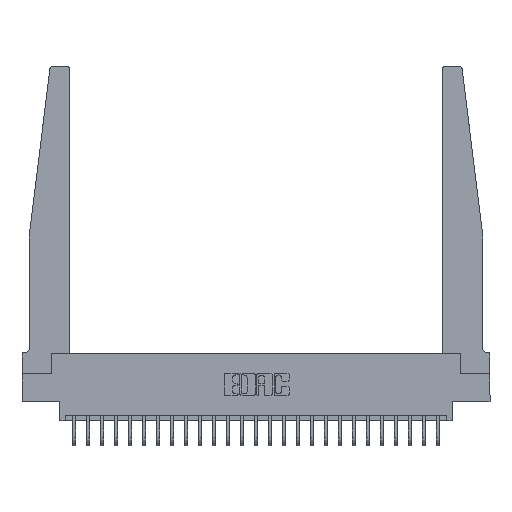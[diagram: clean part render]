
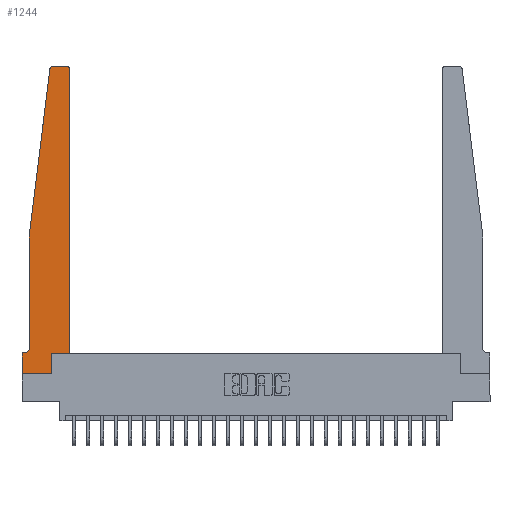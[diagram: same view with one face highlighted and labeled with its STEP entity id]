
A CAD part, top view. The second image highlights one B-rep face of the part: STEP entity #1244.
In plain terms, the highlighted planar face has unit normal (0, 0, 1).
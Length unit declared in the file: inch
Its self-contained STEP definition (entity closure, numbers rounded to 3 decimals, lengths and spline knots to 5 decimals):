
#17 = LINE ( 'NONE', #8325, #12036 ) ;
#75 = VECTOR ( 'NONE', #21901, 39.37008 ) ;
#470 = CARTESIAN_POINT ( 'NONE',  ( 0., 0.1875, 0.37 ) ) ;
#840 = VERTEX_POINT ( 'NONE', #15989 ) ;
#1079 = CARTESIAN_POINT ( 'NONE',  ( 0.015, 0.2375, 0.37 ) ) ;
#1095 = LINE ( 'NONE', #9387, #15164 ) ;
#1244 = ADVANCED_FACE ( 'NONE', ( #25268 ), #2664, .T. ) ;
#1619 = EDGE_CURVE ( 'NONE', #17731, #19536, #25112, .T. ) ;
#2503 = DIRECTION ( 'NONE',  ( 0., 1., 0. ) ) ;
#2549 = CARTESIAN_POINT ( 'NONE',  ( 0.27653, 2.72, 0.37 ) ) ;
#2584 = DIRECTION ( 'NONE',  ( 1., 0., 0. ) ) ;
#2664 = PLANE ( 'NONE',  #6266 ) ;
#2903 = CARTESIAN_POINT ( 'NONE',  ( 0.2605, 0.18, 0.37 ) ) ;
#4219 = AXIS2_PLACEMENT_3D ( 'NONE', #4765, #23035, #2584 ) ;
#4765 = CARTESIAN_POINT ( 'NONE',  ( 0.395, 2.72, 0.37 ) ) ;
#5028 = DIRECTION ( 'NONE',  ( -1., 0., 0. ) ) ;
#5377 = CIRCLE ( 'NONE', #14013, 0.05 ) ;
#5585 = EDGE_CURVE ( 'NONE', #6357, #19973, #24190, .T. ) ;
#5593 = CARTESIAN_POINT ( 'NONE',  ( 0.425, 0.18, 0.37 ) ) ;
#6180 = VERTEX_POINT ( 'NONE', #12797 ) ;
#6217 = ORIENTED_EDGE ( 'NONE', *, *, #12878, .T. ) ;
#6266 = AXIS2_PLACEMENT_3D ( 'NONE', #19333, #17289, #13521 ) ;
#6357 = VERTEX_POINT ( 'NONE', #26037 ) ;
#6876 = EDGE_CURVE ( 'NONE', #20506, #840, #5377, .T. ) ;
#7087 = CARTESIAN_POINT ( 'NONE',  ( 0.065, 0.1875, 0.37 ) ) ;
#7185 = AXIS2_PLACEMENT_3D ( 'NONE', #2549, #10581, #10844 ) ;
#7189 = ORIENTED_EDGE ( 'NONE', *, *, #18088, .T. ) ;
#7559 = CARTESIAN_POINT ( 'NONE',  ( 0.065, 1.25, 0.37 ) ) ;
#8034 = VECTOR ( 'NONE', #17586, 39.37008 ) ;
#8173 = VERTEX_POINT ( 'NONE', #25024 ) ;
#8325 = CARTESIAN_POINT ( 'NONE',  ( 0.25, 2.75, 0.37 ) ) ;
#8416 = EDGE_CURVE ( 'NONE', #6180, #8569, #12769, .T. ) ;
#8569 = VERTEX_POINT ( 'NONE', #12729 ) ;
#8580 = EDGE_CURVE ( 'NONE', #8173, #17731, #17436, .T. ) ;
#9058 = EDGE_CURVE ( 'NONE', #9334, #20506, #13372, .T. ) ;
#9258 = ORIENTED_EDGE ( 'NONE', *, *, #8416, .T. ) ;
#9334 = VERTEX_POINT ( 'NONE', #10247 ) ;
#9387 = CARTESIAN_POINT ( 'NONE',  ( 0.065, 1.25, 0.37 ) ) ;
#9580 = CARTESIAN_POINT ( 'NONE',  ( 0.395, 2.75, 0.37 ) ) ;
#10247 = CARTESIAN_POINT ( 'NONE',  ( 0.065, 1.25, 0.37 ) ) ;
#10307 = ORIENTED_EDGE ( 'NONE', *, *, #8580, .T. ) ;
#10581 = DIRECTION ( 'NONE',  ( 0., 0., 1. ) ) ;
#10647 = ORIENTED_EDGE ( 'NONE', *, *, #6876, .T. ) ;
#10844 = DIRECTION ( 'NONE',  ( 1., 0., 0. ) ) ;
#11281 = EDGE_CURVE ( 'NONE', #840, #21228, #25882, .T. ) ;
#12036 = VECTOR ( 'NONE', #18190, 39.37008 ) ;
#12729 = CARTESIAN_POINT ( 'NONE',  ( 0.24675, 2.72367, 0.37 ) ) ;
#12769 = CIRCLE ( 'NONE', #7185, 0.03 ) ;
#12772 = VECTOR ( 'NONE', #21052, 39.37008 ) ;
#12797 = CARTESIAN_POINT ( 'NONE',  ( 0.27653, 2.75, 0.37 ) ) ;
#12871 = ORIENTED_EDGE ( 'NONE', *, *, #9058, .T. ) ;
#12878 = EDGE_CURVE ( 'NONE', #21324, #6180, #17, .T. ) ;
#12945 = EDGE_CURVE ( 'NONE', #19973, #21324, #20212, .T. ) ;
#13372 = LINE ( 'NONE', #7559, #17549 ) ;
#13521 = DIRECTION ( 'NONE',  ( 1., 0., 0. ) ) ;
#13811 = CARTESIAN_POINT ( 'NONE',  ( 0., 0., 0.37 ) ) ;
#13852 = LINE ( 'NONE', #5593, #23328 ) ;
#14013 = AXIS2_PLACEMENT_3D ( 'NONE', #1079, #26275, #5028 ) ;
#14147 = ORIENTED_EDGE ( 'NONE', *, *, #16750, .T. ) ;
#14499 = EDGE_LOOP ( 'NONE', ( #6217, #9258, #14147, #12871, #10647, #26270, #17759, #10307, #14811, #7189, #22098, #15992 ) ) ;
#14667 = CARTESIAN_POINT ( 'NONE',  ( 0.2605, 0.18, 0.37 ) ) ;
#14811 = ORIENTED_EDGE ( 'NONE', *, *, #1619, .T. ) ;
#14859 = CARTESIAN_POINT ( 'NONE',  ( 0.065, 0.2375, 0.37 ) ) ;
#15164 = VECTOR ( 'NONE', #24103, 39.37008 ) ;
#15989 = CARTESIAN_POINT ( 'NONE',  ( 0.015, 0.1875, 0.37 ) ) ;
#15992 = ORIENTED_EDGE ( 'NONE', *, *, #12945, .T. ) ;
#16750 = EDGE_CURVE ( 'NONE', #8569, #9334, #1095, .T. ) ;
#17004 = CARTESIAN_POINT ( 'NONE',  ( 0., 0., 0.37 ) ) ;
#17289 = DIRECTION ( 'NONE',  ( 0., 0., 1. ) ) ;
#17436 = LINE ( 'NONE', #13811, #8034 ) ;
#17549 = VECTOR ( 'NONE', #23771, 39.37008 ) ;
#17586 = DIRECTION ( 'NONE',  ( 1., 0., 0. ) ) ;
#17731 = VERTEX_POINT ( 'NONE', #20087 ) ;
#17759 = ORIENTED_EDGE ( 'NONE', *, *, #25741, .T. ) ;
#18088 = EDGE_CURVE ( 'NONE', #19536, #6357, #13852, .T. ) ;
#18190 = DIRECTION ( 'NONE',  ( -1., 0., 0. ) ) ;
#19333 = CARTESIAN_POINT ( 'NONE',  ( 0., 0.1875, 0.37 ) ) ;
#19536 = VERTEX_POINT ( 'NONE', #14667 ) ;
#19973 = VERTEX_POINT ( 'NONE', #22867 ) ;
#20087 = CARTESIAN_POINT ( 'NONE',  ( 0.2605, 0., 0.37 ) ) ;
#20137 = CARTESIAN_POINT ( 'NONE',  ( 0.425, 0.18, 0.37 ) ) ;
#20212 = CIRCLE ( 'NONE', #4219, 0.03 ) ;
#20506 = VERTEX_POINT ( 'NONE', #14859 ) ;
#21052 = DIRECTION ( 'NONE',  ( 0., -1., 0. ) ) ;
#21228 = VERTEX_POINT ( 'NONE', #470 ) ;
#21324 = VERTEX_POINT ( 'NONE', #9580 ) ;
#21901 = DIRECTION ( 'NONE',  ( 0., 1., 0. ) ) ;
#22086 = DIRECTION ( 'NONE',  ( 1., 0., 0. ) ) ;
#22098 = ORIENTED_EDGE ( 'NONE', *, *, #5585, .T. ) ;
#22634 = VECTOR ( 'NONE', #2503, 39.37008 ) ;
#22835 = LINE ( 'NONE', #17004, #12772 ) ;
#22867 = CARTESIAN_POINT ( 'NONE',  ( 0.425, 2.72, 0.37 ) ) ;
#23035 = DIRECTION ( 'NONE',  ( 0., 0., 1. ) ) ;
#23328 = VECTOR ( 'NONE', #22086, 39.37008 ) ;
#23570 = DIRECTION ( 'NONE',  ( -1., 0., 0. ) ) ;
#23771 = DIRECTION ( 'NONE',  ( 0., -1., 0. ) ) ;
#24103 = DIRECTION ( 'NONE',  ( -0.122, -0.992, 0. ) ) ;
#24190 = LINE ( 'NONE', #20137, #75 ) ;
#25024 = CARTESIAN_POINT ( 'NONE',  ( 0., 0., 0.37 ) ) ;
#25112 = LINE ( 'NONE', #2903, #22634 ) ;
#25268 = FACE_OUTER_BOUND ( 'NONE', #14499, .T. ) ;
#25319 = VECTOR ( 'NONE', #23570, 39.37008 ) ;
#25741 = EDGE_CURVE ( 'NONE', #21228, #8173, #22835, .T. ) ;
#25882 = LINE ( 'NONE', #7087, #25319 ) ;
#26037 = CARTESIAN_POINT ( 'NONE',  ( 0.425, 0.18, 0.37 ) ) ;
#26270 = ORIENTED_EDGE ( 'NONE', *, *, #11281, .T. ) ;
#26275 = DIRECTION ( 'NONE',  ( 0., 0., -1. ) ) ;
